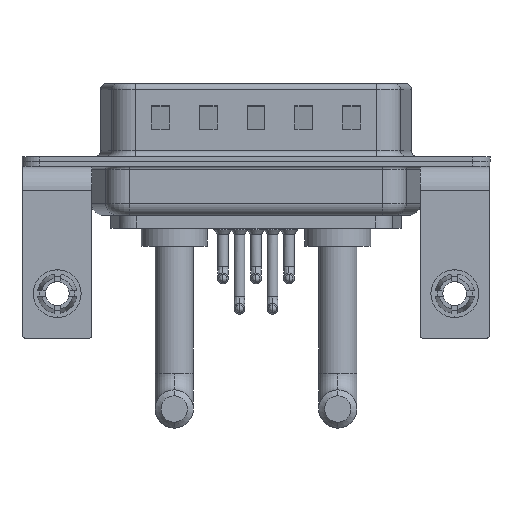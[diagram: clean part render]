
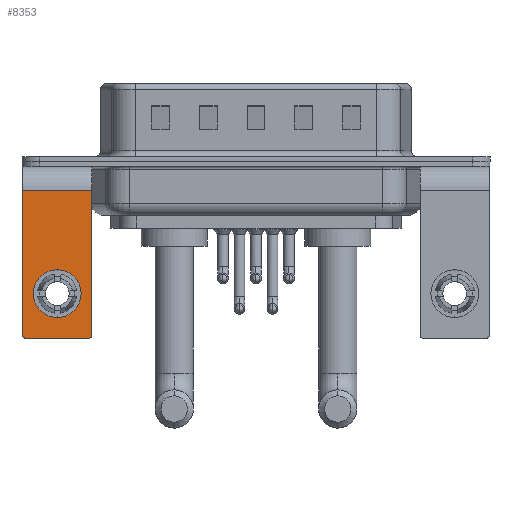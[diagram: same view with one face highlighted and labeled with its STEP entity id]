
A CAD part, front view. The second image highlights one B-rep face of the part: STEP entity #8353.
In plain terms, the highlighted planar face has unit normal (0, -1, 0).
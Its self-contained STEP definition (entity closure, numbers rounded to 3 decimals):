
#211 = DIRECTION ( 'NONE',  ( 0., 1., 0. ) ) ;
#249 = VECTOR ( 'NONE', #3846, 1000. ) ;
#819 = CARTESIAN_POINT ( 'NONE',  ( -2.65, -6.25, -14.8 ) ) ;
#1076 = DIRECTION ( 'NONE',  ( 0., 0., 1. ) ) ;
#1275 = ORIENTED_EDGE ( 'NONE', *, *, #13950, .F. ) ;
#1498 = CARTESIAN_POINT ( 'NONE',  ( -2.9, -6.25, -2.4 ) ) ;
#2038 = EDGE_CURVE ( 'NONE', #2835, #8618, #7583, .T. ) ;
#2108 = ORIENTED_EDGE ( 'NONE', *, *, #20117, .T. ) ;
#2277 = VERTEX_POINT ( 'NONE', #11460 ) ;
#2835 = VERTEX_POINT ( 'NONE', #3722 ) ;
#3347 = EDGE_CURVE ( 'NONE', #8753, #16575, #14532, .T. ) ;
#3722 = CARTESIAN_POINT ( 'NONE',  ( -2.9, -6.25, -14.55 ) ) ;
#3782 = CARTESIAN_POINT ( 'NONE',  ( 2.9, -6.25, -2.4 ) ) ;
#3815 = CARTESIAN_POINT ( 'NONE',  ( 0., -6.25, -13.07 ) ) ;
#3846 = DIRECTION ( 'NONE',  ( -1., 0., 0. ) ) ;
#4425 = ORIENTED_EDGE ( 'NONE', *, *, #3347, .F. ) ;
#4601 = DIRECTION ( 'NONE',  ( 0., 1., 0. ) ) ;
#5464 = LINE ( 'NONE', #23299, #11910 ) ;
#6271 = CARTESIAN_POINT ( 'NONE',  ( 0., -6.25, -9.07 ) ) ;
#6368 = ORIENTED_EDGE ( 'NONE', *, *, #18656, .T. ) ;
#6648 = EDGE_CURVE ( 'NONE', #14489, #2835, #19833, .T. ) ;
#7583 = CIRCLE ( 'NONE', #10603, 0.25 ) ;
#8353 = ADVANCED_FACE ( 'NONE', ( #18996, #10030 ), #13687, .F. ) ;
#8618 = VERTEX_POINT ( 'NONE', #819 ) ;
#8753 = VERTEX_POINT ( 'NONE', #20278 ) ;
#8984 = DIRECTION ( 'NONE',  ( 0., 0., 1. ) ) ;
#10030 = FACE_OUTER_BOUND ( 'NONE', #13441, .T. ) ;
#10035 = AXIS2_PLACEMENT_3D ( 'NONE', #22759, #211, #14603 ) ;
#10603 = AXIS2_PLACEMENT_3D ( 'NONE', #14185, #19846, #8984 ) ;
#10793 = DIRECTION ( 'NONE',  ( -1., 0., 0. ) ) ;
#10948 = CARTESIAN_POINT ( 'NONE',  ( 2.9, -6.25, -14.8 ) ) ;
#11170 = EDGE_LOOP ( 'NONE', ( #6368, #15444 ) ) ;
#11460 = CARTESIAN_POINT ( 'NONE',  ( 2.65, -6.25, -14.8 ) ) ;
#11910 = VECTOR ( 'NONE', #10793, 1000. ) ;
#12020 = EDGE_CURVE ( 'NONE', #2277, #16575, #19453, .T. ) ;
#12843 = ORIENTED_EDGE ( 'NONE', *, *, #2038, .T. ) ;
#13255 = VERTEX_POINT ( 'NONE', #3815 ) ;
#13441 = EDGE_LOOP ( 'NONE', ( #18756, #12843, #1275, #20918, #4425, #2108 ) ) ;
#13687 = PLANE ( 'NONE',  #18461 ) ;
#13906 = EDGE_CURVE ( 'NONE', #22017, #13255, #18331, .T. ) ;
#13950 = EDGE_CURVE ( 'NONE', #2277, #8618, #18026, .T. ) ;
#14082 = DIRECTION ( 'NONE',  ( 0., 0., 1. ) ) ;
#14125 = AXIS2_PLACEMENT_3D ( 'NONE', #14891, #16791, #20328 ) ;
#14185 = CARTESIAN_POINT ( 'NONE',  ( -2.65, -6.25, -14.55 ) ) ;
#14305 = DIRECTION ( 'NONE',  ( 0., 0., -1. ) ) ;
#14322 = DIRECTION ( 'NONE',  ( 0., -1., 0. ) ) ;
#14489 = VERTEX_POINT ( 'NONE', #1498 ) ;
#14532 = LINE ( 'NONE', #3782, #19217 ) ;
#14603 = DIRECTION ( 'NONE',  ( 0., 0., 1. ) ) ;
#14891 = CARTESIAN_POINT ( 'NONE',  ( 0., -6.25, -11.07 ) ) ;
#15444 = ORIENTED_EDGE ( 'NONE', *, *, #13906, .T. ) ;
#15568 = CARTESIAN_POINT ( 'NONE',  ( 2.9, -6.25, -2.4 ) ) ;
#16175 = CARTESIAN_POINT ( 'NONE',  ( -2.9, -6.25, -2.4 ) ) ;
#16291 = DIRECTION ( 'NONE',  ( 0., 0., -1. ) ) ;
#16575 = VERTEX_POINT ( 'NONE', #22847 ) ;
#16791 = DIRECTION ( 'NONE',  ( 0., 1., 0. ) ) ;
#18026 = LINE ( 'NONE', #10948, #249 ) ;
#18331 = CIRCLE ( 'NONE', #10035, 2. ) ;
#18461 = AXIS2_PLACEMENT_3D ( 'NONE', #15568, #4601, #1076 ) ;
#18656 = EDGE_CURVE ( 'NONE', #13255, #22017, #20897, .T. ) ;
#18756 = ORIENTED_EDGE ( 'NONE', *, *, #6648, .T. ) ;
#18996 = FACE_BOUND ( 'NONE', #11170, .T. ) ;
#19217 = VECTOR ( 'NONE', #14305, 1000. ) ;
#19453 = CIRCLE ( 'NONE', #21696, 0.25 ) ;
#19833 = LINE ( 'NONE', #16175, #21472 ) ;
#19846 = DIRECTION ( 'NONE',  ( 0., -1., 0. ) ) ;
#20117 = EDGE_CURVE ( 'NONE', #8753, #14489, #5464, .T. ) ;
#20278 = CARTESIAN_POINT ( 'NONE',  ( 2.9, -6.25, -2.4 ) ) ;
#20328 = DIRECTION ( 'NONE',  ( 0., 0., 1. ) ) ;
#20897 = CIRCLE ( 'NONE', #14125, 2. ) ;
#20918 = ORIENTED_EDGE ( 'NONE', *, *, #12020, .T. ) ;
#21472 = VECTOR ( 'NONE', #16291, 1000. ) ;
#21516 = CARTESIAN_POINT ( 'NONE',  ( 2.65, -6.25, -14.55 ) ) ;
#21696 = AXIS2_PLACEMENT_3D ( 'NONE', #21516, #14322, #14082 ) ;
#22017 = VERTEX_POINT ( 'NONE', #6271 ) ;
#22759 = CARTESIAN_POINT ( 'NONE',  ( 0., -6.25, -11.07 ) ) ;
#22847 = CARTESIAN_POINT ( 'NONE',  ( 2.9, -6.25, -14.55 ) ) ;
#23299 = CARTESIAN_POINT ( 'NONE',  ( 2.9, -6.25, -2.4 ) ) ;
